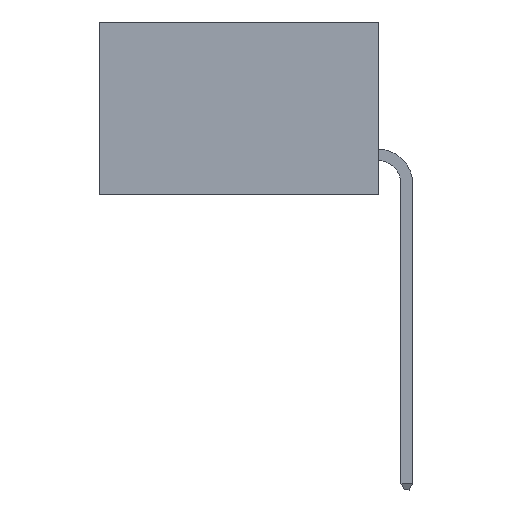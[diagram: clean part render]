
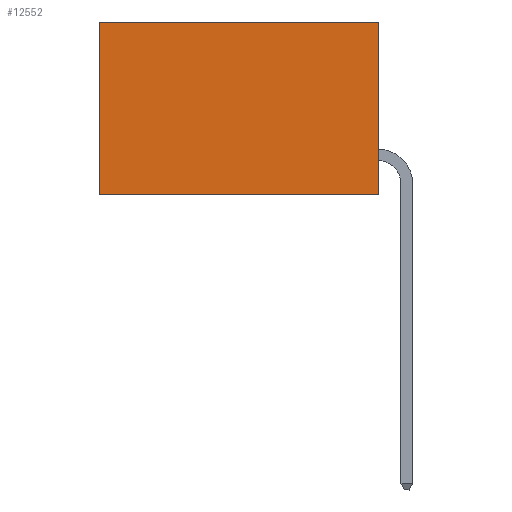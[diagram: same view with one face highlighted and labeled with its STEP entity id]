
A CAD part, left-side view. The second image highlights one B-rep face of the part: STEP entity #12552.
In plain terms, the highlighted planar face has unit normal (-1, 0, 0).
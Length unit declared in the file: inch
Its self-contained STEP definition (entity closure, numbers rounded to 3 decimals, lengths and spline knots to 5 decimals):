
#515 = DIRECTION ( 'NONE',  ( 0., 1., 0. ) ) ;
#1809 = LINE ( 'NONE', #15422, #19075 ) ;
#1813 = FACE_OUTER_BOUND ( 'NONE', #15573, .T. ) ;
#2002 = CARTESIAN_POINT ( 'NONE',  ( 0.2615, 0., -0.37 ) ) ;
#2012 = DIRECTION ( 'NONE',  ( 0., 0., -1. ) ) ;
#2177 = CARTESIAN_POINT ( 'NONE',  ( 0.2615, 0., 0. ) ) ;
#3540 = LINE ( 'NONE', #2177, #17557 ) ;
#3599 = CARTESIAN_POINT ( 'NONE',  ( 0.2615, 0., -0.37 ) ) ;
#3976 = AXIS2_PLACEMENT_3D ( 'NONE', #13948, #9497, #16979 ) ;
#5507 = VERTEX_POINT ( 'NONE', #14780 ) ;
#6169 = EDGE_CURVE ( 'NONE', #5507, #17039, #1809, .T. ) ;
#7401 = EDGE_CURVE ( 'NONE', #13906, #5507, #3540, .T. ) ;
#7902 = ORIENTED_EDGE ( 'NONE', *, *, #18531, .F. ) ;
#8131 = CARTESIAN_POINT ( 'NONE',  ( 0.2615, 0., 0. ) ) ;
#9086 = ORIENTED_EDGE ( 'NONE', *, *, #14426, .F. ) ;
#9484 = DIRECTION ( 'NONE',  ( 0., 1., 0. ) ) ;
#9497 = DIRECTION ( 'NONE',  ( 1., 0., 0. ) ) ;
#10645 = CARTESIAN_POINT ( 'NONE',  ( 0.2615, 0., -0.37 ) ) ;
#10751 = CARTESIAN_POINT ( 'NONE',  ( 0.2615, 0.6, -0.37 ) ) ;
#10860 = PLANE ( 'NONE',  #3976 ) ;
#12552 = ADVANCED_FACE ( 'NONE', ( #1813 ), #10860, .F. ) ;
#12958 = DIRECTION ( 'NONE',  ( 0., 0., -1. ) ) ;
#13239 = ORIENTED_EDGE ( 'NONE', *, *, #6169, .T. ) ;
#13906 = VERTEX_POINT ( 'NONE', #8131 ) ;
#13926 = LINE ( 'NONE', #10645, #17088 ) ;
#13948 = CARTESIAN_POINT ( 'NONE',  ( 0.2615, 0., -0.37 ) ) ;
#14130 = LINE ( 'NONE', #2002, #17466 ) ;
#14426 = EDGE_CURVE ( 'NONE', #13906, #17555, #13926, .T. ) ;
#14661 = ORIENTED_EDGE ( 'NONE', *, *, #7401, .T. ) ;
#14780 = CARTESIAN_POINT ( 'NONE',  ( 0.2615, 0.6, 0. ) ) ;
#15422 = CARTESIAN_POINT ( 'NONE',  ( 0.2615, 0.6, -0.37 ) ) ;
#15573 = EDGE_LOOP ( 'NONE', ( #13239, #7902, #9086, #14661 ) ) ;
#16979 = DIRECTION ( 'NONE',  ( 0., 0., -1. ) ) ;
#17039 = VERTEX_POINT ( 'NONE', #10751 ) ;
#17088 = VECTOR ( 'NONE', #12958, 39.37008 ) ;
#17466 = VECTOR ( 'NONE', #9484, 39.37008 ) ;
#17555 = VERTEX_POINT ( 'NONE', #3599 ) ;
#17557 = VECTOR ( 'NONE', #515, 39.37008 ) ;
#18531 = EDGE_CURVE ( 'NONE', #17555, #17039, #14130, .T. ) ;
#19075 = VECTOR ( 'NONE', #2012, 39.37008 ) ;
